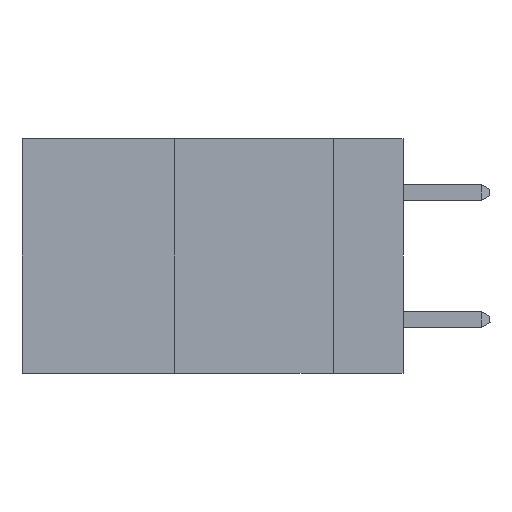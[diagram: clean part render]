
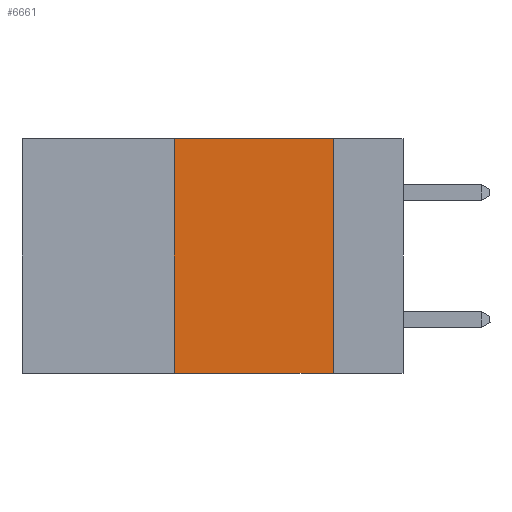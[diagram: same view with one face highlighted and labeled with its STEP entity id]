
A CAD part, left-side view. The second image highlights one B-rep face of the part: STEP entity #6661.
In plain terms, the highlighted planar face has unit normal (-1, 0, 0).
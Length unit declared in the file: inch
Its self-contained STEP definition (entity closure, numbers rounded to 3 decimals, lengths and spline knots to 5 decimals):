
#589 = CARTESIAN_POINT ( 'NONE',  ( 0., 0.6, 0. ) ) ;
#599 = EDGE_CURVE ( 'NONE', #4445, #6622, #7033, .T. ) ;
#861 = CARTESIAN_POINT ( 'NONE',  ( 0., 0.6, -0.37 ) ) ;
#1083 = CARTESIAN_POINT ( 'NONE',  ( 0., 0.6, 0. ) ) ;
#1618 = EDGE_LOOP ( 'NONE', ( #8357, #5056, #6712, #7966 ) ) ;
#1781 = AXIS2_PLACEMENT_3D ( 'NONE', #1083, #4602, #5281 ) ;
#1849 = CARTESIAN_POINT ( 'NONE',  ( 0., 0.11, 0. ) ) ;
#2052 = FACE_OUTER_BOUND ( 'NONE', #1618, .T. ) ;
#2409 = CARTESIAN_POINT ( 'NONE',  ( 0., 0.36, 0. ) ) ;
#2491 = DIRECTION ( 'NONE',  ( 0., 0., 1. ) ) ;
#3080 = CARTESIAN_POINT ( 'NONE',  ( 0., 0.11, 0. ) ) ;
#3131 = CARTESIAN_POINT ( 'NONE',  ( 0., 0.36, 0. ) ) ;
#3243 = VERTEX_POINT ( 'NONE', #5081 ) ;
#3283 = DIRECTION ( 'NONE',  ( 0., 0., -1. ) ) ;
#3578 = LINE ( 'NONE', #1849, #5290 ) ;
#3780 = CARTESIAN_POINT ( 'NONE',  ( 0., 0.36, -0.37 ) ) ;
#4392 = LINE ( 'NONE', #861, #6551 ) ;
#4445 = VERTEX_POINT ( 'NONE', #2409 ) ;
#4578 = PLANE ( 'NONE',  #1781 ) ;
#4602 = DIRECTION ( 'NONE',  ( 1., 0., 0. ) ) ;
#4660 = EDGE_CURVE ( 'NONE', #5077, #3243, #4392, .T. ) ;
#5056 = ORIENTED_EDGE ( 'NONE', *, *, #599, .F. ) ;
#5077 = VERTEX_POINT ( 'NONE', #3780 ) ;
#5081 = CARTESIAN_POINT ( 'NONE',  ( 0., 0.11, -0.37 ) ) ;
#5281 = DIRECTION ( 'NONE',  ( 0., 0., -1. ) ) ;
#5290 = VECTOR ( 'NONE', #3283, 39.37008 ) ;
#5593 = VECTOR ( 'NONE', #7520, 39.37008 ) ;
#6423 = EDGE_CURVE ( 'NONE', #6622, #3243, #3578, .T. ) ;
#6487 = DIRECTION ( 'NONE',  ( 0., -1., 0. ) ) ;
#6551 = VECTOR ( 'NONE', #6487, 39.37008 ) ;
#6622 = VERTEX_POINT ( 'NONE', #3080 ) ;
#6661 = ADVANCED_FACE ( 'NONE', ( #2052 ), #4578, .F. ) ;
#6712 = ORIENTED_EDGE ( 'NONE', *, *, #7057, .F. ) ;
#7033 = LINE ( 'NONE', #589, #5593 ) ;
#7057 = EDGE_CURVE ( 'NONE', #5077, #4445, #8365, .T. ) ;
#7520 = DIRECTION ( 'NONE',  ( 0., -1., 0. ) ) ;
#7926 = VECTOR ( 'NONE', #2491, 39.37008 ) ;
#7966 = ORIENTED_EDGE ( 'NONE', *, *, #4660, .T. ) ;
#8357 = ORIENTED_EDGE ( 'NONE', *, *, #6423, .F. ) ;
#8365 = LINE ( 'NONE', #3131, #7926 ) ;
